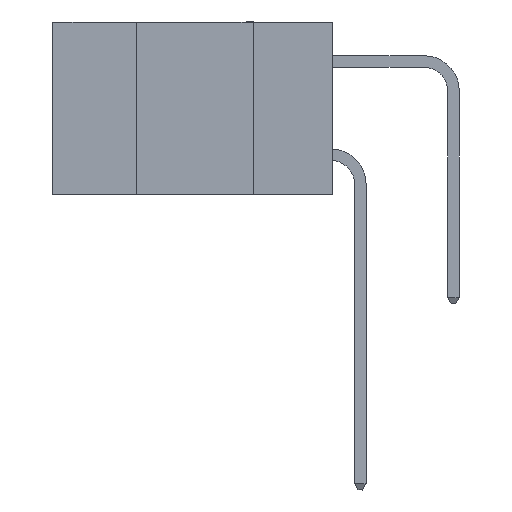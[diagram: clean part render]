
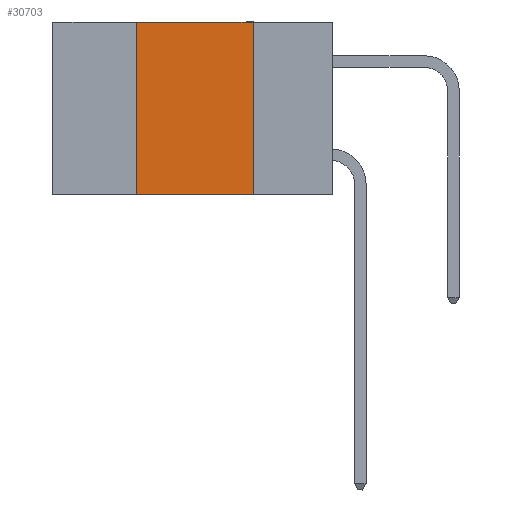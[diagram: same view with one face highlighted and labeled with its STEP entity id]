
A CAD part, left-side view. The second image highlights one B-rep face of the part: STEP entity #30703.
In plain terms, the highlighted planar face has unit normal (-1, 0, 0).
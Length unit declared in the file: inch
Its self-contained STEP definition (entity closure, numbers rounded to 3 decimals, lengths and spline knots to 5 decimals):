
#574 = ORIENTED_EDGE ( 'NONE', *, *, #24239, .F. ) ;
#1539 = FACE_OUTER_BOUND ( 'NONE', #27714, .T. ) ;
#4096 = DIRECTION ( 'NONE',  ( 0., -1., 0. ) ) ;
#4190 = CARTESIAN_POINT ( 'NONE',  ( 0., 0.17, 0. ) ) ;
#5077 = VERTEX_POINT ( 'NONE', #4190 ) ;
#6224 = DIRECTION ( 'NONE',  ( 0., -1., 0. ) ) ;
#6602 = VECTOR ( 'NONE', #6224, 39.37008 ) ;
#7367 = VECTOR ( 'NONE', #21713, 39.37008 ) ;
#8390 = PLANE ( 'NONE',  #11761 ) ;
#10130 = VERTEX_POINT ( 'NONE', #32284 ) ;
#10246 = VECTOR ( 'NONE', #15899, 39.37008 ) ;
#11020 = CARTESIAN_POINT ( 'NONE',  ( 0., 0.6, 0. ) ) ;
#11761 = AXIS2_PLACEMENT_3D ( 'NONE', #11020, #13630, #31845 ) ;
#12620 = EDGE_CURVE ( 'NONE', #5077, #10130, #30233, .T. ) ;
#12853 = CARTESIAN_POINT ( 'NONE',  ( 0., 0.42, 0. ) ) ;
#13630 = DIRECTION ( 'NONE',  ( 1., 0., 0. ) ) ;
#14144 = VERTEX_POINT ( 'NONE', #21739 ) ;
#15899 = DIRECTION ( 'NONE',  ( 0., 0., -1. ) ) ;
#16713 = CARTESIAN_POINT ( 'NONE',  ( 0., 0.6, 0. ) ) ;
#18682 = EDGE_CURVE ( 'NONE', #21341, #5077, #27417, .T. ) ;
#19085 = CARTESIAN_POINT ( 'NONE',  ( 0., 0.42, 0. ) ) ;
#19706 = ORIENTED_EDGE ( 'NONE', *, *, #12620, .F. ) ;
#19708 = CARTESIAN_POINT ( 'NONE',  ( 0., 0.6, -0.37 ) ) ;
#20085 = EDGE_CURVE ( 'NONE', #14144, #10130, #27645, .T. ) ;
#21253 = LINE ( 'NONE', #19085, #7367 ) ;
#21341 = VERTEX_POINT ( 'NONE', #12853 ) ;
#21713 = DIRECTION ( 'NONE',  ( 0., 0., 1. ) ) ;
#21739 = CARTESIAN_POINT ( 'NONE',  ( 0., 0.42, -0.37 ) ) ;
#24239 = EDGE_CURVE ( 'NONE', #14144, #21341, #21253, .T. ) ;
#27417 = LINE ( 'NONE', #16713, #6602 ) ;
#27645 = LINE ( 'NONE', #19708, #29298 ) ;
#27714 = EDGE_LOOP ( 'NONE', ( #19706, #27953, #574, #33711 ) ) ;
#27953 = ORIENTED_EDGE ( 'NONE', *, *, #18682, .F. ) ;
#29298 = VECTOR ( 'NONE', #4096, 39.37008 ) ;
#30233 = LINE ( 'NONE', #31523, #10246 ) ;
#30703 = ADVANCED_FACE ( 'NONE', ( #1539 ), #8390, .F. ) ;
#31523 = CARTESIAN_POINT ( 'NONE',  ( 0., 0.17, 0. ) ) ;
#31845 = DIRECTION ( 'NONE',  ( 0., 0., -1. ) ) ;
#32284 = CARTESIAN_POINT ( 'NONE',  ( 0., 0.17, -0.37 ) ) ;
#33711 = ORIENTED_EDGE ( 'NONE', *, *, #20085, .T. ) ;
